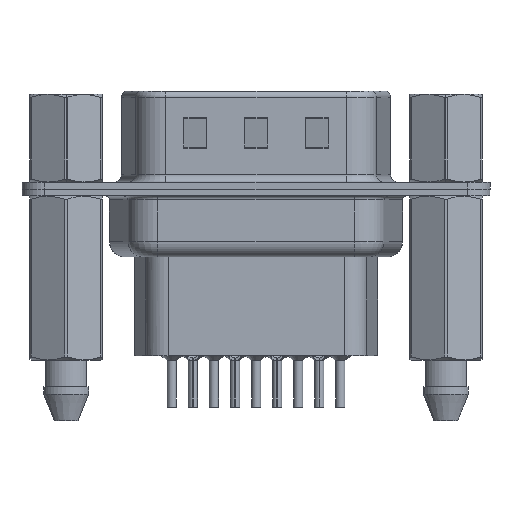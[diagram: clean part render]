
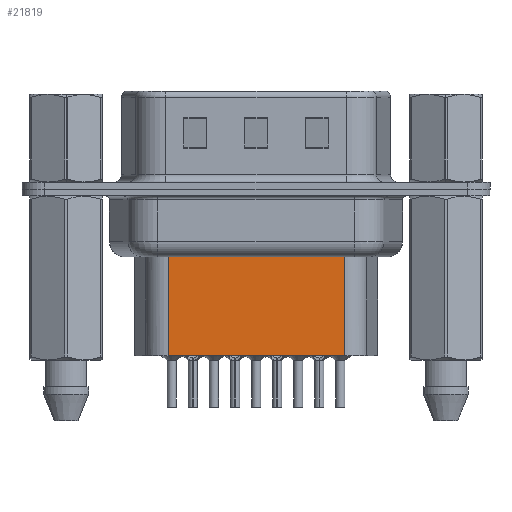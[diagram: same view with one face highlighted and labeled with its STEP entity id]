
A CAD part, front view. The second image highlights one B-rep face of the part: STEP entity #21819.
In plain terms, the highlighted planar face has unit normal (0, -1, 0).
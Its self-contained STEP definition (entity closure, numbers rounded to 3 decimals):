
#404 = DIRECTION ( 'NONE',  ( 0., 0., -1. ) ) ;
#723 = CARTESIAN_POINT ( 'NONE',  ( 18.294, -3.5, -4.097 ) ) ;
#803 = LINE ( 'NONE', #2993, #11347 ) ;
#901 = CARTESIAN_POINT ( 'NONE',  ( 6.706, -3.5, -3.1 ) ) ;
#922 = DIRECTION ( 'NONE',  ( -1., 0., 0. ) ) ;
#2304 = VERTEX_POINT ( 'NONE', #20965 ) ;
#2442 = LINE ( 'NONE', #10817, #12550 ) ;
#2688 = CARTESIAN_POINT ( 'NONE',  ( 6.459, -3.5, -4.097 ) ) ;
#2856 = DIRECTION ( 'NONE',  ( 0., 0., -1. ) ) ;
#2906 = VECTOR ( 'NONE', #922, 1000. ) ;
#2993 = CARTESIAN_POINT ( 'NONE',  ( 18.294, -3.5, -3.1 ) ) ;
#3341 = LINE ( 'NONE', #26126, #15801 ) ;
#4315 = VERTEX_POINT ( 'NONE', #11035 ) ;
#5399 = DIRECTION ( 'NONE',  ( -1., 0., 0. ) ) ;
#6563 = EDGE_CURVE ( 'NONE', #17015, #22601, #17648, .T. ) ;
#6907 = PLANE ( 'NONE',  #11762 ) ;
#7273 = EDGE_CURVE ( 'NONE', #4315, #2304, #3341, .T. ) ;
#8061 = EDGE_LOOP ( 'NONE', ( #8433, #23802, #9149, #18594 ) ) ;
#8433 = ORIENTED_EDGE ( 'NONE', *, *, #8736, .F. ) ;
#8736 = EDGE_CURVE ( 'NONE', #17015, #4315, #803, .T. ) ;
#9149 = ORIENTED_EDGE ( 'NONE', *, *, #25372, .T. ) ;
#10817 = CARTESIAN_POINT ( 'NONE',  ( 6.706, -3.5, -3.1 ) ) ;
#11035 = CARTESIAN_POINT ( 'NONE',  ( 18.294, -3.5, -10.95 ) ) ;
#11305 = FACE_OUTER_BOUND ( 'NONE', #8061, .T. ) ;
#11347 = VECTOR ( 'NONE', #2856, 1000. ) ;
#11488 = CARTESIAN_POINT ( 'NONE',  ( 6.706, -3.5, -4.097 ) ) ;
#11581 = DIRECTION ( 'NONE',  ( 0., -1., 0. ) ) ;
#11762 = AXIS2_PLACEMENT_3D ( 'NONE', #901, #11581, #19698 ) ;
#12550 = VECTOR ( 'NONE', #404, 1000. ) ;
#15801 = VECTOR ( 'NONE', #5399, 1000. ) ;
#17015 = VERTEX_POINT ( 'NONE', #723 ) ;
#17648 = LINE ( 'NONE', #2688, #2906 ) ;
#18594 = ORIENTED_EDGE ( 'NONE', *, *, #7273, .F. ) ;
#19698 = DIRECTION ( 'NONE',  ( 1., 0., 0. ) ) ;
#20965 = CARTESIAN_POINT ( 'NONE',  ( 6.706, -3.5, -10.95 ) ) ;
#21819 = ADVANCED_FACE ( 'NONE', ( #11305 ), #6907, .T. ) ;
#22601 = VERTEX_POINT ( 'NONE', #11488 ) ;
#23802 = ORIENTED_EDGE ( 'NONE', *, *, #6563, .T. ) ;
#25372 = EDGE_CURVE ( 'NONE', #22601, #2304, #2442, .T. ) ;
#26126 = CARTESIAN_POINT ( 'NONE',  ( 6.706, -3.5, -10.95 ) ) ;
